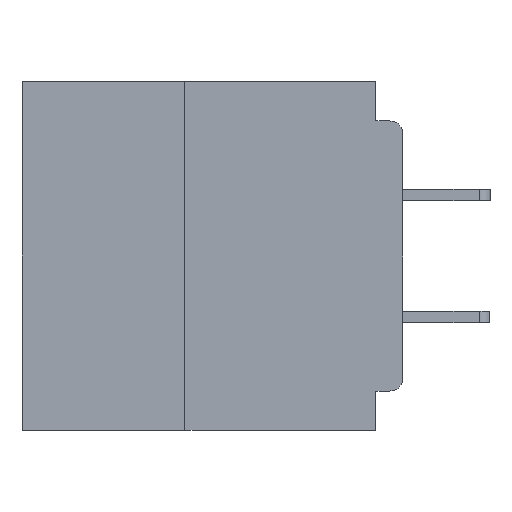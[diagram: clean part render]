
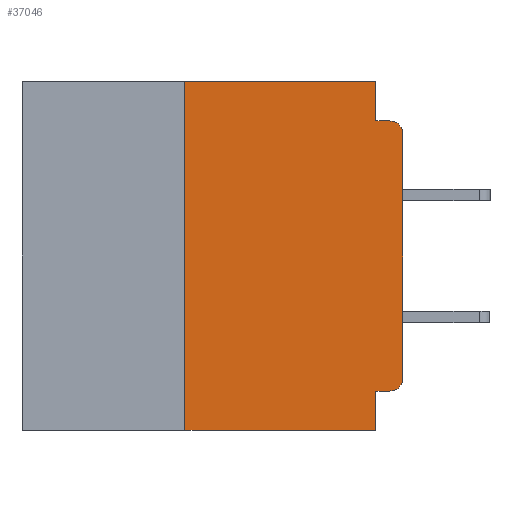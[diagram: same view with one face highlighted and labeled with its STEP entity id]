
A CAD part, left-side view. The second image highlights one B-rep face of the part: STEP entity #37046.
In plain terms, the highlighted planar face has unit normal (-1, 0, 0).
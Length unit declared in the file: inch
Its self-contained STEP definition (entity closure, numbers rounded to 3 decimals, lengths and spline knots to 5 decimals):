
#100 = VECTOR ( 'NONE', #32062, 39.37008 ) ;
#983 = DIRECTION ( 'NONE',  ( 0., 1., 0. ) ) ;
#2320 = CARTESIAN_POINT ( 'NONE',  ( 0., 0.437, 0. ) ) ;
#2415 = AXIS2_PLACEMENT_3D ( 'NONE', #2320, #32388, #6665 ) ;
#2591 = EDGE_CURVE ( 'NONE', #33330, #44461, #32040, .T. ) ;
#2764 = DIRECTION ( 'NONE',  ( 0., 0., -1. ) ) ;
#3218 = VERTEX_POINT ( 'NONE', #26117 ) ;
#4496 = CARTESIAN_POINT ( 'NONE',  ( 0., 0.031, 0. ) ) ;
#4662 = CARTESIAN_POINT ( 'NONE',  ( 0., 0.437, 0. ) ) ;
#5225 = EDGE_CURVE ( 'NONE', #33073, #6501, #45187, .T. ) ;
#6501 = VERTEX_POINT ( 'NONE', #8226 ) ;
#6665 = DIRECTION ( 'NONE',  ( 0., 0., -1. ) ) ;
#7482 = CARTESIAN_POINT ( 'NONE',  ( 0., 0.015, -0.34 ) ) ;
#7681 = VERTEX_POINT ( 'NONE', #15790 ) ;
#8226 = CARTESIAN_POINT ( 'NONE',  ( 0., 0.25, 0. ) ) ;
#9920 = VECTOR ( 'NONE', #35573, 39.37008 ) ;
#10045 = AXIS2_PLACEMENT_3D ( 'NONE', #42677, #16993, #46992 ) ;
#10926 = VECTOR ( 'NONE', #52232, 39.37008 ) ;
#11504 = LINE ( 'NONE', #14768, #100 ) ;
#11773 = DIRECTION ( 'NONE',  ( 0., 0., -1. ) ) ;
#12592 = ORIENTED_EDGE ( 'NONE', *, *, #14189, .F. ) ;
#13077 = ORIENTED_EDGE ( 'NONE', *, *, #48599, .F. ) ;
#14014 = CARTESIAN_POINT ( 'NONE',  ( 0., 0.031, 0. ) ) ;
#14189 = EDGE_CURVE ( 'NONE', #25392, #45199, #43166, .T. ) ;
#14768 = CARTESIAN_POINT ( 'NONE',  ( 0., 0.437, -0.4 ) ) ;
#15790 = CARTESIAN_POINT ( 'NONE',  ( 0., 0., -0.06 ) ) ;
#16993 = DIRECTION ( 'NONE',  ( -1., 0., 0. ) ) ;
#17486 = LINE ( 'NONE', #31145, #48990 ) ;
#20675 = CARTESIAN_POINT ( 'NONE',  ( 0., 0.031, -0.4 ) ) ;
#22975 = VERTEX_POINT ( 'NONE', #53168 ) ;
#23743 = PLANE ( 'NONE',  #2415 ) ;
#25392 = VERTEX_POINT ( 'NONE', #47765 ) ;
#26074 = DIRECTION ( 'NONE',  ( 0., -1., 0. ) ) ;
#26117 = CARTESIAN_POINT ( 'NONE',  ( 0., 0.015, -0.045 ) ) ;
#26423 = CARTESIAN_POINT ( 'NONE',  ( 0., 0.25, -0.4 ) ) ;
#26819 = ORIENTED_EDGE ( 'NONE', *, *, #29017, .F. ) ;
#27966 = ORIENTED_EDGE ( 'NONE', *, *, #37552, .F. ) ;
#28631 = LINE ( 'NONE', #48100, #50032 ) ;
#29017 = EDGE_CURVE ( 'NONE', #6501, #33330, #34113, .T. ) ;
#29842 = CARTESIAN_POINT ( 'NONE',  ( 0., 0.25, -0.4 ) ) ;
#30443 = VECTOR ( 'NONE', #50648, 39.37008 ) ;
#30702 = VECTOR ( 'NONE', #2764, 39.37008 ) ;
#31107 = ORIENTED_EDGE ( 'NONE', *, *, #35315, .T. ) ;
#31145 = CARTESIAN_POINT ( 'NONE',  ( 0., 0., 0. ) ) ;
#31217 = CIRCLE ( 'NONE', #47190, 0.015 ) ;
#32040 = LINE ( 'NONE', #4496, #30702 ) ;
#32062 = DIRECTION ( 'NONE',  ( 0., -1., 0. ) ) ;
#32388 = DIRECTION ( 'NONE',  ( 1., 0., 0. ) ) ;
#32784 = LINE ( 'NONE', #48423, #9920 ) ;
#33073 = VERTEX_POINT ( 'NONE', #29842 ) ;
#33330 = VERTEX_POINT ( 'NONE', #14014 ) ;
#33690 = CARTESIAN_POINT ( 'NONE',  ( 0., 0.031, -0.045 ) ) ;
#34113 = LINE ( 'NONE', #4662, #45471 ) ;
#34146 = EDGE_LOOP ( 'NONE', ( #35993, #37238, #27966, #49857, #26819, #44538, #31107, #12592, #13077, #54003 ) ) ;
#35315 = EDGE_CURVE ( 'NONE', #33073, #45199, #11504, .T. ) ;
#35573 = DIRECTION ( 'NONE',  ( 0., -1., 0. ) ) ;
#35993 = ORIENTED_EDGE ( 'NONE', *, *, #36359, .T. ) ;
#36359 = EDGE_CURVE ( 'NONE', #22975, #7681, #17486, .T. ) ;
#36915 = FACE_OUTER_BOUND ( 'NONE', #34146, .T. ) ;
#37046 = ADVANCED_FACE ( 'NONE', ( #36915 ), #23743, .F. ) ;
#37238 = ORIENTED_EDGE ( 'NONE', *, *, #42380, .T. ) ;
#37552 = EDGE_CURVE ( 'NONE', #44461, #3218, #32784, .T. ) ;
#37581 = DIRECTION ( 'NONE',  ( -1., 0., 0. ) ) ;
#37775 = VERTEX_POINT ( 'NONE', #50072 ) ;
#38351 = CARTESIAN_POINT ( 'NONE',  ( 0., 0.031, -0.4 ) ) ;
#39413 = DIRECTION ( 'NONE',  ( 0., 0., 1. ) ) ;
#42380 = EDGE_CURVE ( 'NONE', #7681, #3218, #54733, .T. ) ;
#42677 = CARTESIAN_POINT ( 'NONE',  ( 0., 0.015, -0.06 ) ) ;
#43166 = LINE ( 'NONE', #20675, #30443 ) ;
#44461 = VERTEX_POINT ( 'NONE', #33690 ) ;
#44538 = ORIENTED_EDGE ( 'NONE', *, *, #5225, .F. ) ;
#45187 = LINE ( 'NONE', #26423, #10926 ) ;
#45199 = VERTEX_POINT ( 'NONE', #38351 ) ;
#45471 = VECTOR ( 'NONE', #26074, 39.37008 ) ;
#46992 = DIRECTION ( 'NONE',  ( 0., 0., -1. ) ) ;
#47190 = AXIS2_PLACEMENT_3D ( 'NONE', #7482, #37581, #11773 ) ;
#47765 = CARTESIAN_POINT ( 'NONE',  ( 0., 0.031, -0.355 ) ) ;
#48100 = CARTESIAN_POINT ( 'NONE',  ( 0., 0., -0.355 ) ) ;
#48423 = CARTESIAN_POINT ( 'NONE',  ( 0., 0., -0.045 ) ) ;
#48599 = EDGE_CURVE ( 'NONE', #37775, #25392, #28631, .T. ) ;
#48990 = VECTOR ( 'NONE', #39413, 39.37008 ) ;
#49857 = ORIENTED_EDGE ( 'NONE', *, *, #2591, .F. ) ;
#50032 = VECTOR ( 'NONE', #983, 39.37008 ) ;
#50072 = CARTESIAN_POINT ( 'NONE',  ( 0., 0.015, -0.355 ) ) ;
#50648 = DIRECTION ( 'NONE',  ( 0., 0., -1. ) ) ;
#52232 = DIRECTION ( 'NONE',  ( 0., 0., 1. ) ) ;
#53168 = CARTESIAN_POINT ( 'NONE',  ( 0., 0., -0.34 ) ) ;
#54003 = ORIENTED_EDGE ( 'NONE', *, *, #55447, .T. ) ;
#54733 = CIRCLE ( 'NONE', #10045, 0.015 ) ;
#55447 = EDGE_CURVE ( 'NONE', #37775, #22975, #31217, .T. ) ;
